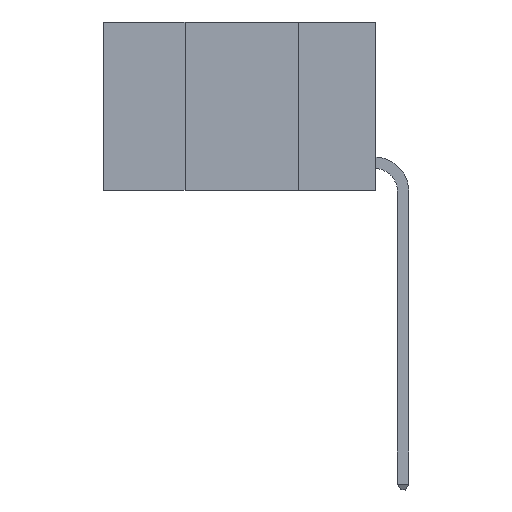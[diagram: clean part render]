
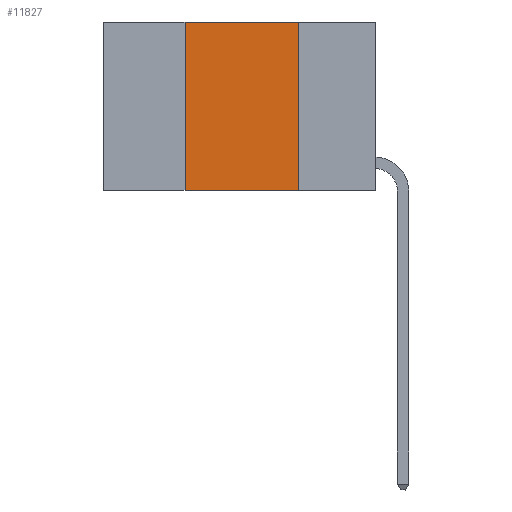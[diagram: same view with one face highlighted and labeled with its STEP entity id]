
A CAD part, left-side view. The second image highlights one B-rep face of the part: STEP entity #11827.
In plain terms, the highlighted planar face has unit normal (-1, 0, 0).
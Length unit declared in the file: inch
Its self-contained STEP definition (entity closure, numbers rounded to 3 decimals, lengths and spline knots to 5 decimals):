
#90 = CARTESIAN_POINT ( 'NONE',  ( 0., 0.6, -0.37 ) ) ;
#168 = AXIS2_PLACEMENT_3D ( 'NONE', #4925, #13583, #6158 ) ;
#362 = FACE_OUTER_BOUND ( 'NONE', #5166, .T. ) ;
#1086 = VERTEX_POINT ( 'NONE', #11197 ) ;
#1662 = DIRECTION ( 'NONE',  ( 0., 0., -1. ) ) ;
#1712 = VERTEX_POINT ( 'NONE', #9753 ) ;
#2376 = DIRECTION ( 'NONE',  ( 0., -1., 0. ) ) ;
#3955 = ORIENTED_EDGE ( 'NONE', *, *, #7966, .T. ) ;
#3987 = VERTEX_POINT ( 'NONE', #12370 ) ;
#4799 = CARTESIAN_POINT ( 'NONE',  ( 0., 0.6, 0. ) ) ;
#4925 = CARTESIAN_POINT ( 'NONE',  ( 0., 0.6, 0. ) ) ;
#5166 = EDGE_LOOP ( 'NONE', ( #8378, #10259, #8128, #3955 ) ) ;
#5186 = VECTOR ( 'NONE', #1662, 39.37008 ) ;
#5282 = VECTOR ( 'NONE', #6762, 39.37008 ) ;
#5549 = EDGE_CURVE ( 'NONE', #1712, #14363, #8855, .T. ) ;
#6158 = DIRECTION ( 'NONE',  ( 0., 0., -1. ) ) ;
#6762 = DIRECTION ( 'NONE',  ( 0., 0., 1. ) ) ;
#6953 = VECTOR ( 'NONE', #2376, 39.37008 ) ;
#7836 = CARTESIAN_POINT ( 'NONE',  ( 0., 0.17, 0. ) ) ;
#7966 = EDGE_CURVE ( 'NONE', #1086, #14363, #15533, .T. ) ;
#8128 = ORIENTED_EDGE ( 'NONE', *, *, #8410, .F. ) ;
#8378 = ORIENTED_EDGE ( 'NONE', *, *, #5549, .F. ) ;
#8410 = EDGE_CURVE ( 'NONE', #1086, #3987, #8564, .T. ) ;
#8564 = LINE ( 'NONE', #15388, #5282 ) ;
#8783 = DIRECTION ( 'NONE',  ( 0., -1., 0. ) ) ;
#8855 = LINE ( 'NONE', #7836, #5186 ) ;
#9753 = CARTESIAN_POINT ( 'NONE',  ( 0., 0.17, 0. ) ) ;
#10222 = CARTESIAN_POINT ( 'NONE',  ( 0., 0.17, -0.37 ) ) ;
#10259 = ORIENTED_EDGE ( 'NONE', *, *, #13750, .F. ) ;
#10281 = LINE ( 'NONE', #4799, #6953 ) ;
#11197 = CARTESIAN_POINT ( 'NONE',  ( 0., 0.42, -0.37 ) ) ;
#11827 = ADVANCED_FACE ( 'NONE', ( #362 ), #12351, .F. ) ;
#11885 = VECTOR ( 'NONE', #8783, 39.37008 ) ;
#12351 = PLANE ( 'NONE',  #168 ) ;
#12370 = CARTESIAN_POINT ( 'NONE',  ( 0., 0.42, 0. ) ) ;
#13583 = DIRECTION ( 'NONE',  ( 1., 0., 0. ) ) ;
#13750 = EDGE_CURVE ( 'NONE', #3987, #1712, #10281, .T. ) ;
#14363 = VERTEX_POINT ( 'NONE', #10222 ) ;
#15388 = CARTESIAN_POINT ( 'NONE',  ( 0., 0.42, 0. ) ) ;
#15533 = LINE ( 'NONE', #90, #11885 ) ;
